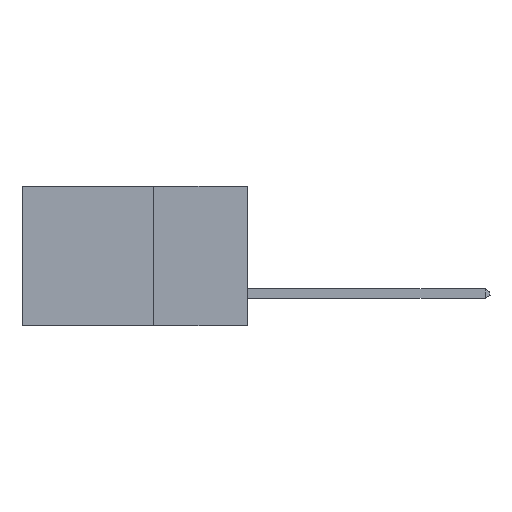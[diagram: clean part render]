
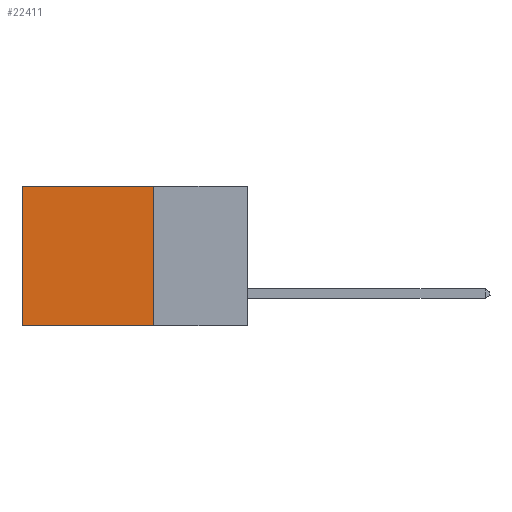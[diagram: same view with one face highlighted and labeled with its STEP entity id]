
A CAD part, left-side view. The second image highlights one B-rep face of the part: STEP entity #22411.
In plain terms, the highlighted planar face has unit normal (-1, 0, 0).
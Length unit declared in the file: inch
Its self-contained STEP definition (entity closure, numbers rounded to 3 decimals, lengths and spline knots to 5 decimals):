
#120 = CARTESIAN_POINT ( 'NONE',  ( 0.298, 0.6, 0. ) ) ;
#1377 = VECTOR ( 'NONE', #21489, 39.37008 ) ;
#1387 = CARTESIAN_POINT ( 'NONE',  ( 0.298, 0.25, 0. ) ) ;
#1522 = VECTOR ( 'NONE', #7554, 39.37008 ) ;
#2368 = VERTEX_POINT ( 'NONE', #120 ) ;
#3394 = ORIENTED_EDGE ( 'NONE', *, *, #10241, .T. ) ;
#3705 = VERTEX_POINT ( 'NONE', #17177 ) ;
#4167 = FACE_OUTER_BOUND ( 'NONE', #18575, .T. ) ;
#5686 = ORIENTED_EDGE ( 'NONE', *, *, #14347, .F. ) ;
#5878 = CARTESIAN_POINT ( 'NONE',  ( 0.298, 0.25, -0.37 ) ) ;
#6901 = VECTOR ( 'NONE', #13579, 39.37008 ) ;
#7554 = DIRECTION ( 'NONE',  ( 0., 0., -1. ) ) ;
#7872 = EDGE_CURVE ( 'NONE', #17451, #12641, #17216, .T. ) ;
#8138 = ORIENTED_EDGE ( 'NONE', *, *, #22349, .T. ) ;
#10029 = AXIS2_PLACEMENT_3D ( 'NONE', #20911, #20983, #12201 ) ;
#10241 = EDGE_CURVE ( 'NONE', #2368, #3705, #22327, .T. ) ;
#10357 = PLANE ( 'NONE',  #10029 ) ;
#10475 = CARTESIAN_POINT ( 'NONE',  ( 0.298, 0.25, 0. ) ) ;
#10916 = CARTESIAN_POINT ( 'NONE',  ( 0.298, 0.6, 0. ) ) ;
#11831 = VECTOR ( 'NONE', #16738, 39.37008 ) ;
#12201 = DIRECTION ( 'NONE',  ( 0., 0., -1. ) ) ;
#12641 = VERTEX_POINT ( 'NONE', #5878 ) ;
#12778 = ORIENTED_EDGE ( 'NONE', *, *, #7872, .F. ) ;
#13579 = DIRECTION ( 'NONE',  ( 0., 1., 0. ) ) ;
#14347 = EDGE_CURVE ( 'NONE', #12641, #3705, #22545, .T. ) ;
#16738 = DIRECTION ( 'NONE',  ( 0., 1., 0. ) ) ;
#17177 = CARTESIAN_POINT ( 'NONE',  ( 0.298, 0.6, -0.37 ) ) ;
#17216 = LINE ( 'NONE', #19415, #1377 ) ;
#17451 = VERTEX_POINT ( 'NONE', #10475 ) ;
#18185 = CARTESIAN_POINT ( 'NONE',  ( 0.298, 0.25, -0.37 ) ) ;
#18575 = EDGE_LOOP ( 'NONE', ( #3394, #5686, #12778, #8138 ) ) ;
#19415 = CARTESIAN_POINT ( 'NONE',  ( 0.298, 0.25, 0. ) ) ;
#20901 = LINE ( 'NONE', #1387, #6901 ) ;
#20911 = CARTESIAN_POINT ( 'NONE',  ( 0.298, 0.25, 0. ) ) ;
#20983 = DIRECTION ( 'NONE',  ( 1., 0., 0. ) ) ;
#21489 = DIRECTION ( 'NONE',  ( 0., 0., -1. ) ) ;
#22327 = LINE ( 'NONE', #10916, #1522 ) ;
#22349 = EDGE_CURVE ( 'NONE', #17451, #2368, #20901, .T. ) ;
#22411 = ADVANCED_FACE ( 'NONE', ( #4167 ), #10357, .F. ) ;
#22545 = LINE ( 'NONE', #18185, #11831 ) ;
